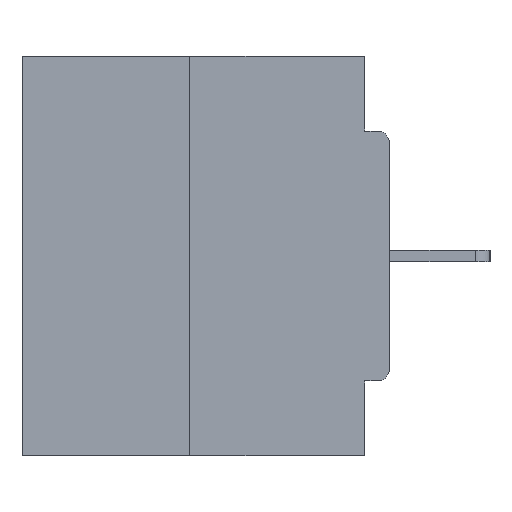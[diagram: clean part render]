
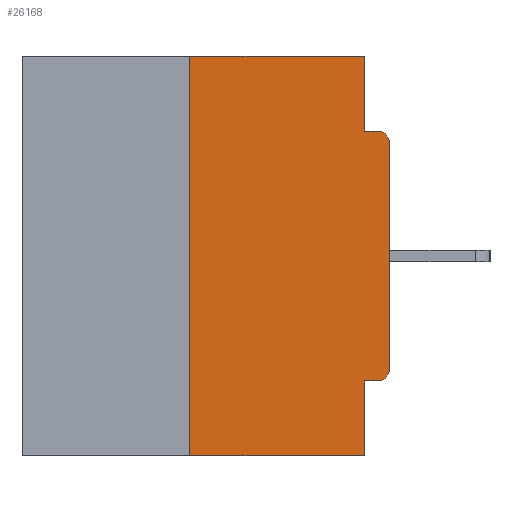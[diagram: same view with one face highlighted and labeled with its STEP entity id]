
A CAD part, left-side view. The second image highlights one B-rep face of the part: STEP entity #26168.
In plain terms, the highlighted planar face has unit normal (-1, 0, 0).
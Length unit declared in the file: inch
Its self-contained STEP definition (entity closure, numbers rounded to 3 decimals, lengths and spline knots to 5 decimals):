
#387 = VERTEX_POINT ( 'NONE', #26351 ) ;
#1271 = ORIENTED_EDGE ( 'NONE', *, *, #28621, .F. ) ;
#1309 = DIRECTION ( 'NONE',  ( 0., -1., 0. ) ) ;
#2611 = EDGE_CURVE ( 'NONE', #12042, #387, #25039, .T. ) ;
#3149 = DIRECTION ( 'NONE',  ( 0., -1., 0. ) ) ;
#3335 = DIRECTION ( 'NONE',  ( 0., -1., 0. ) ) ;
#3602 = CARTESIAN_POINT ( 'NONE',  ( 0., 0.46, 0. ) ) ;
#3639 = LINE ( 'NONE', #22589, #27127 ) ;
#3805 = ORIENTED_EDGE ( 'NONE', *, *, #30225, .T. ) ;
#4032 = CARTESIAN_POINT ( 'NONE',  ( 0., 0.031, -0.5 ) ) ;
#4361 = FACE_OUTER_BOUND ( 'NONE', #27088, .T. ) ;
#4626 = VERTEX_POINT ( 'NONE', #17691 ) ;
#4858 = CARTESIAN_POINT ( 'NONE',  ( 0., 0.25, 0. ) ) ;
#5953 = VECTOR ( 'NONE', #3149, 39.37008 ) ;
#6151 = VERTEX_POINT ( 'NONE', #29021 ) ;
#6455 = DIRECTION ( 'NONE',  ( -1., 0., 0. ) ) ;
#7066 = VECTOR ( 'NONE', #12570, 39.37008 ) ;
#7777 = LINE ( 'NONE', #12738, #9941 ) ;
#8871 = CARTESIAN_POINT ( 'NONE',  ( 0., 0.46, 0. ) ) ;
#8903 = EDGE_CURVE ( 'NONE', #19441, #26605, #3639, .T. ) ;
#9332 = DIRECTION ( 'NONE',  ( 1., 0., 0. ) ) ;
#9394 = ORIENTED_EDGE ( 'NONE', *, *, #19367, .F. ) ;
#9571 = CARTESIAN_POINT ( 'NONE',  ( 0., 0.031, -0.0935 ) ) ;
#9941 = VECTOR ( 'NONE', #17688, 39.37008 ) ;
#11343 = PLANE ( 'NONE',  #28904 ) ;
#11645 = ORIENTED_EDGE ( 'NONE', *, *, #8903, .F. ) ;
#11698 = DIRECTION ( 'NONE',  ( -1., 0., 0. ) ) ;
#12042 = VERTEX_POINT ( 'NONE', #26704 ) ;
#12556 = ORIENTED_EDGE ( 'NONE', *, *, #17991, .F. ) ;
#12570 = DIRECTION ( 'NONE',  ( 0., 1., 0. ) ) ;
#12738 = CARTESIAN_POINT ( 'NONE',  ( 0., 0.031, -0.5 ) ) ;
#12806 = CARTESIAN_POINT ( 'NONE',  ( 0., 0.46, -0.5 ) ) ;
#12978 = VECTOR ( 'NONE', #25580, 39.37008 ) ;
#13008 = VERTEX_POINT ( 'NONE', #4032 ) ;
#13509 = CARTESIAN_POINT ( 'NONE',  ( 0., 0., -0.3915 ) ) ;
#14512 = AXIS2_PLACEMENT_3D ( 'NONE', #21493, #11698, #28778 ) ;
#15436 = AXIS2_PLACEMENT_3D ( 'NONE', #27725, #6455, #18390 ) ;
#16154 = DIRECTION ( 'NONE',  ( 0., 0., -1. ) ) ;
#16570 = DIRECTION ( 'NONE',  ( 0., 0., 1. ) ) ;
#16994 = EDGE_CURVE ( 'NONE', #26325, #20658, #27911, .T. ) ;
#16997 = EDGE_CURVE ( 'NONE', #4626, #12042, #21169, .T. ) ;
#17688 = DIRECTION ( 'NONE',  ( 0., 0., -1. ) ) ;
#17691 = CARTESIAN_POINT ( 'NONE',  ( 0., 0.25, -0.5 ) ) ;
#17991 = EDGE_CURVE ( 'NONE', #26325, #27923, #19709, .T. ) ;
#18390 = DIRECTION ( 'NONE',  ( 0., 0., -1. ) ) ;
#18471 = VECTOR ( 'NONE', #30639, 39.37008 ) ;
#18615 = CARTESIAN_POINT ( 'NONE',  ( 0., 0.015, -0.0935 ) ) ;
#18955 = VECTOR ( 'NONE', #16570, 39.37008 ) ;
#19226 = ORIENTED_EDGE ( 'NONE', *, *, #27938, .T. ) ;
#19367 = EDGE_CURVE ( 'NONE', #387, #19441, #30218, .T. ) ;
#19441 = VERTEX_POINT ( 'NONE', #9571 ) ;
#19709 = LINE ( 'NONE', #26706, #7066 ) ;
#20658 = VERTEX_POINT ( 'NONE', #13509 ) ;
#21087 = LINE ( 'NONE', #28691, #18955 ) ;
#21169 = LINE ( 'NONE', #4858, #18471 ) ;
#21493 = CARTESIAN_POINT ( 'NONE',  ( 0., 0.015, -0.3915 ) ) ;
#22589 = CARTESIAN_POINT ( 'NONE',  ( 0., 0., -0.0935 ) ) ;
#22897 = CIRCLE ( 'NONE', #15436, 0.015 ) ;
#24470 = LINE ( 'NONE', #12806, #29832 ) ;
#25039 = LINE ( 'NONE', #3602, #5953 ) ;
#25580 = DIRECTION ( 'NONE',  ( 0., 0., -1. ) ) ;
#25809 = ORIENTED_EDGE ( 'NONE', *, *, #16994, .T. ) ;
#26168 = ADVANCED_FACE ( 'NONE', ( #4361 ), #11343, .F. ) ;
#26189 = CARTESIAN_POINT ( 'NONE',  ( 0., 0.031, 0. ) ) ;
#26325 = VERTEX_POINT ( 'NONE', #26890 ) ;
#26351 = CARTESIAN_POINT ( 'NONE',  ( 0., 0.031, 0. ) ) ;
#26605 = VERTEX_POINT ( 'NONE', #18615 ) ;
#26704 = CARTESIAN_POINT ( 'NONE',  ( 0., 0.25, 0. ) ) ;
#26706 = CARTESIAN_POINT ( 'NONE',  ( 0., 0., -0.4065 ) ) ;
#26890 = CARTESIAN_POINT ( 'NONE',  ( 0., 0.015, -0.4065 ) ) ;
#27088 = EDGE_LOOP ( 'NONE', ( #30417, #28048, #30031, #1271, #12556, #25809, #3805, #19226, #11645, #9394 ) ) ;
#27127 = VECTOR ( 'NONE', #1309, 39.37008 ) ;
#27442 = CARTESIAN_POINT ( 'NONE',  ( 0., 0.031, -0.4065 ) ) ;
#27725 = CARTESIAN_POINT ( 'NONE',  ( 0., 0.015, -0.1085 ) ) ;
#27911 = CIRCLE ( 'NONE', #14512, 0.015 ) ;
#27923 = VERTEX_POINT ( 'NONE', #27442 ) ;
#27938 = EDGE_CURVE ( 'NONE', #6151, #26605, #22897, .T. ) ;
#28048 = ORIENTED_EDGE ( 'NONE', *, *, #16997, .F. ) ;
#28621 = EDGE_CURVE ( 'NONE', #27923, #13008, #7777, .T. ) ;
#28691 = CARTESIAN_POINT ( 'NONE',  ( 0., 0., 0. ) ) ;
#28778 = DIRECTION ( 'NONE',  ( 0., 0., -1. ) ) ;
#28904 = AXIS2_PLACEMENT_3D ( 'NONE', #8871, #9332, #16154 ) ;
#29021 = CARTESIAN_POINT ( 'NONE',  ( 0., 0., -0.1085 ) ) ;
#29473 = EDGE_CURVE ( 'NONE', #4626, #13008, #24470, .T. ) ;
#29832 = VECTOR ( 'NONE', #3335, 39.37008 ) ;
#30031 = ORIENTED_EDGE ( 'NONE', *, *, #29473, .T. ) ;
#30218 = LINE ( 'NONE', #26189, #12978 ) ;
#30225 = EDGE_CURVE ( 'NONE', #20658, #6151, #21087, .T. ) ;
#30417 = ORIENTED_EDGE ( 'NONE', *, *, #2611, .F. ) ;
#30639 = DIRECTION ( 'NONE',  ( 0., 0., 1. ) ) ;
